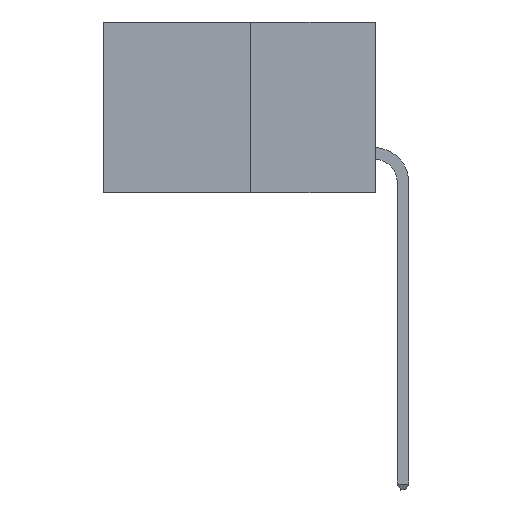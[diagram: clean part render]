
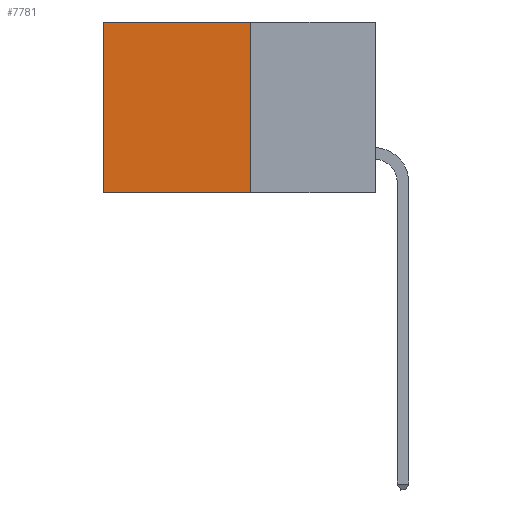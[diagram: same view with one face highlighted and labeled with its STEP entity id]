
A CAD part, left-side view. The second image highlights one B-rep face of the part: STEP entity #7781.
In plain terms, the highlighted planar face has unit normal (-1, 0, 0).
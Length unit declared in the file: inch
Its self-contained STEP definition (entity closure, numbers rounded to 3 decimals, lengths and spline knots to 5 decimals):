
#3 = CARTESIAN_POINT ( 'NONE',  ( 0.277, 0.27, 0. ) ) ;
#432 = EDGE_CURVE ( 'NONE', #6675, #7946, #6960, .T. ) ;
#846 = ORIENTED_EDGE ( 'NONE', *, *, #4061, .F. ) ;
#1118 = LINE ( 'NONE', #2519, #8790 ) ;
#1468 = DIRECTION ( 'NONE',  ( 0., 1., 0. ) ) ;
#2519 = CARTESIAN_POINT ( 'NONE',  ( 0.277, 0.27, -0.37 ) ) ;
#2568 = VECTOR ( 'NONE', #1468, 39.37008 ) ;
#2793 = CARTESIAN_POINT ( 'NONE',  ( 0.277, 0.59, 0. ) ) ;
#2893 = LINE ( 'NONE', #2919, #8413 ) ;
#2919 = CARTESIAN_POINT ( 'NONE',  ( 0.277, 0.27, -0.37 ) ) ;
#3046 = DIRECTION ( 'NONE',  ( 0., 0., -1. ) ) ;
#3190 = EDGE_CURVE ( 'NONE', #6675, #4542, #2893, .T. ) ;
#3757 = VECTOR ( 'NONE', #5486, 39.37008 ) ;
#3839 = VERTEX_POINT ( 'NONE', #4606 ) ;
#4061 = EDGE_CURVE ( 'NONE', #4542, #3839, #1118, .T. ) ;
#4220 = DIRECTION ( 'NONE',  ( 0., 0., -1. ) ) ;
#4253 = DIRECTION ( 'NONE',  ( 1., 0., 0. ) ) ;
#4278 = PLANE ( 'NONE',  #5983 ) ;
#4347 = CARTESIAN_POINT ( 'NONE',  ( 0.277, 0.27, -0.37 ) ) ;
#4409 = CARTESIAN_POINT ( 'NONE',  ( 0.277, 0.27, 0. ) ) ;
#4542 = VERTEX_POINT ( 'NONE', #6898 ) ;
#4606 = CARTESIAN_POINT ( 'NONE',  ( 0.277, 0.59, -0.37 ) ) ;
#4866 = ORIENTED_EDGE ( 'NONE', *, *, #432, .T. ) ;
#5486 = DIRECTION ( 'NONE',  ( 0., 0., -1. ) ) ;
#5983 = AXIS2_PLACEMENT_3D ( 'NONE', #4347, #4253, #4220 ) ;
#6369 = EDGE_LOOP ( 'NONE', ( #8080, #846, #8826, #4866 ) ) ;
#6675 = VERTEX_POINT ( 'NONE', #3 ) ;
#6818 = FACE_OUTER_BOUND ( 'NONE', #6369, .T. ) ;
#6898 = CARTESIAN_POINT ( 'NONE',  ( 0.277, 0.27, -0.37 ) ) ;
#6938 = EDGE_CURVE ( 'NONE', #7946, #3839, #9147, .T. ) ;
#6960 = LINE ( 'NONE', #4409, #2568 ) ;
#7537 = CARTESIAN_POINT ( 'NONE',  ( 0.277, 0.59, -0.37 ) ) ;
#7781 = ADVANCED_FACE ( 'NONE', ( #6818 ), #4278, .F. ) ;
#7946 = VERTEX_POINT ( 'NONE', #2793 ) ;
#8080 = ORIENTED_EDGE ( 'NONE', *, *, #6938, .T. ) ;
#8413 = VECTOR ( 'NONE', #3046, 39.37008 ) ;
#8790 = VECTOR ( 'NONE', #9576, 39.37008 ) ;
#8826 = ORIENTED_EDGE ( 'NONE', *, *, #3190, .F. ) ;
#9147 = LINE ( 'NONE', #7537, #3757 ) ;
#9576 = DIRECTION ( 'NONE',  ( 0., 1., 0. ) ) ;
